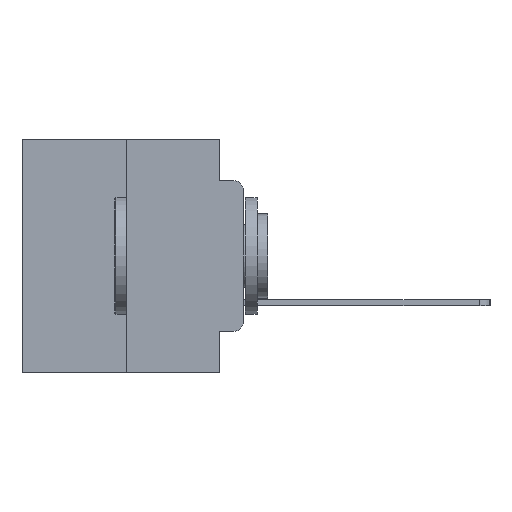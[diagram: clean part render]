
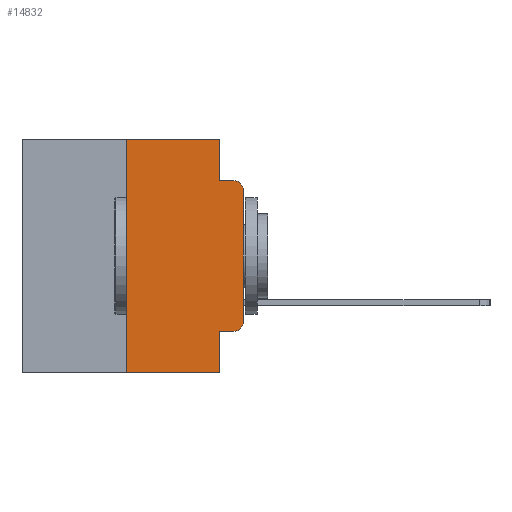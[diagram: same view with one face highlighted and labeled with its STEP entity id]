
A CAD part, left-side view. The second image highlights one B-rep face of the part: STEP entity #14832.
In plain terms, the highlighted planar face has unit normal (-1, 0, 0).
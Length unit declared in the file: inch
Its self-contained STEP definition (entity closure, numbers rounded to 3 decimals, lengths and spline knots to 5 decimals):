
#293 = DIRECTION ( 'NONE',  ( 0., -1., 0. ) ) ;
#563 = DIRECTION ( 'NONE',  ( 0., 0., -1. ) ) ;
#1384 = ORIENTED_EDGE ( 'NONE', *, *, #14961, .F. ) ;
#1643 = LINE ( 'NONE', #5594, #18598 ) ;
#1685 = LINE ( 'NONE', #14650, #23465 ) ;
#1740 = EDGE_CURVE ( 'NONE', #13574, #17665, #1643, .T. ) ;
#1890 = DIRECTION ( 'NONE',  ( 0., -1., 0. ) ) ;
#2057 = VECTOR ( 'NONE', #2701, 39.37008 ) ;
#2079 = CARTESIAN_POINT ( 'NONE',  ( 0., 0.051, -0.4115 ) ) ;
#2270 = CARTESIAN_POINT ( 'NONE',  ( 0., 0., 0. ) ) ;
#2387 = DIRECTION ( 'NONE',  ( 0., -1., 0. ) ) ;
#2701 = DIRECTION ( 'NONE',  ( 0., 0., -1. ) ) ;
#3762 = CARTESIAN_POINT ( 'NONE',  ( 0., 0., -0.1085 ) ) ;
#3891 = DIRECTION ( 'NONE',  ( 0., 0., 1. ) ) ;
#4120 = DIRECTION ( 'NONE',  ( 0., -1., 0. ) ) ;
#4228 = CARTESIAN_POINT ( 'NONE',  ( 0., 0.051, 0. ) ) ;
#4357 = CARTESIAN_POINT ( 'NONE',  ( 0., 0.051, 0. ) ) ;
#5004 = FACE_OUTER_BOUND ( 'NONE', #26360, .T. ) ;
#5014 = ORIENTED_EDGE ( 'NONE', *, *, #18480, .T. ) ;
#5594 = CARTESIAN_POINT ( 'NONE',  ( 0., 0.473, -0.5 ) ) ;
#5695 = ORIENTED_EDGE ( 'NONE', *, *, #17080, .T. ) ;
#5769 = CARTESIAN_POINT ( 'NONE',  ( 0., 0.051, -0.5 ) ) ;
#5929 = VERTEX_POINT ( 'NONE', #19667 ) ;
#6376 = ORIENTED_EDGE ( 'NONE', *, *, #14221, .F. ) ;
#7090 = EDGE_CURVE ( 'NONE', #27107, #26037, #23311, .T. ) ;
#7099 = CARTESIAN_POINT ( 'NONE',  ( 0., 0.02, -0.1085 ) ) ;
#7884 = PLANE ( 'NONE',  #15399 ) ;
#8397 = ORIENTED_EDGE ( 'NONE', *, *, #9958, .F. ) ;
#8549 = EDGE_CURVE ( 'NONE', #12620, #27107, #23541, .T. ) ;
#8835 = AXIS2_PLACEMENT_3D ( 'NONE', #7099, #21842, #9261 ) ;
#9261 = DIRECTION ( 'NONE',  ( 0., 0., -1. ) ) ;
#9958 = EDGE_CURVE ( 'NONE', #12620, #17665, #11955, .T. ) ;
#11428 = VECTOR ( 'NONE', #3891, 39.37008 ) ;
#11955 = LINE ( 'NONE', #4228, #22459 ) ;
#12131 = CARTESIAN_POINT ( 'NONE',  ( 0., 0.473, 0. ) ) ;
#12415 = VECTOR ( 'NONE', #4120, 39.37008 ) ;
#12528 = CARTESIAN_POINT ( 'NONE',  ( 0., 0.25, 0. ) ) ;
#12605 = CARTESIAN_POINT ( 'NONE',  ( 0., 0.02, -0.4115 ) ) ;
#12620 = VERTEX_POINT ( 'NONE', #24255 ) ;
#12792 = EDGE_CURVE ( 'NONE', #13574, #22755, #17098, .T. ) ;
#13329 = DIRECTION ( 'NONE',  ( -1., 0., 0. ) ) ;
#13376 = LINE ( 'NONE', #15489, #2057 ) ;
#13574 = VERTEX_POINT ( 'NONE', #23852 ) ;
#14066 = LINE ( 'NONE', #15180, #19654 ) ;
#14221 = EDGE_CURVE ( 'NONE', #19597, #5929, #13376, .T. ) ;
#14277 = DIRECTION ( 'NONE',  ( 0., 0., -1. ) ) ;
#14650 = CARTESIAN_POINT ( 'NONE',  ( 0., 0.473, 0. ) ) ;
#14832 = ADVANCED_FACE ( 'NONE', ( #5004 ), #7884, .F. ) ;
#14866 = DIRECTION ( 'NONE',  ( 0., 0., -1. ) ) ;
#14961 = EDGE_CURVE ( 'NONE', #22755, #19597, #1685, .T. ) ;
#15180 = CARTESIAN_POINT ( 'NONE',  ( 0., 0.051, -0.0885 ) ) ;
#15399 = AXIS2_PLACEMENT_3D ( 'NONE', #12131, #26707, #14277 ) ;
#15489 = CARTESIAN_POINT ( 'NONE',  ( 0., 0.051, 0. ) ) ;
#15669 = EDGE_CURVE ( 'NONE', #5929, #20698, #14066, .T. ) ;
#17036 = ORIENTED_EDGE ( 'NONE', *, *, #15669, .F. ) ;
#17080 = EDGE_CURVE ( 'NONE', #20389, #20698, #23771, .T. ) ;
#17098 = LINE ( 'NONE', #26942, #11428 ) ;
#17184 = DIRECTION ( 'NONE',  ( 0., 0., 1. ) ) ;
#17665 = VERTEX_POINT ( 'NONE', #5769 ) ;
#18275 = AXIS2_PLACEMENT_3D ( 'NONE', #25791, #13329, #563 ) ;
#18480 = EDGE_CURVE ( 'NONE', #26037, #20389, #19818, .T. ) ;
#18598 = VECTOR ( 'NONE', #293, 39.37008 ) ;
#18994 = ORIENTED_EDGE ( 'NONE', *, *, #1740, .T. ) ;
#19597 = VERTEX_POINT ( 'NONE', #4357 ) ;
#19624 = ORIENTED_EDGE ( 'NONE', *, *, #8549, .T. ) ;
#19654 = VECTOR ( 'NONE', #2387, 39.37008 ) ;
#19667 = CARTESIAN_POINT ( 'NONE',  ( 0., 0.051, -0.0885 ) ) ;
#19818 = LINE ( 'NONE', #2270, #25295 ) ;
#20389 = VERTEX_POINT ( 'NONE', #3762 ) ;
#20698 = VERTEX_POINT ( 'NONE', #21672 ) ;
#21672 = CARTESIAN_POINT ( 'NONE',  ( 0., 0.02, -0.0885 ) ) ;
#21842 = DIRECTION ( 'NONE',  ( -1., 0., 0. ) ) ;
#22459 = VECTOR ( 'NONE', #14866, 39.37008 ) ;
#22755 = VERTEX_POINT ( 'NONE', #12528 ) ;
#23311 = CIRCLE ( 'NONE', #18275, 0.02 ) ;
#23465 = VECTOR ( 'NONE', #1890, 39.37008 ) ;
#23541 = LINE ( 'NONE', #2079, #12415 ) ;
#23771 = CIRCLE ( 'NONE', #8835, 0.02 ) ;
#23804 = CARTESIAN_POINT ( 'NONE',  ( 0., 0., -0.3915 ) ) ;
#23810 = ORIENTED_EDGE ( 'NONE', *, *, #12792, .F. ) ;
#23852 = CARTESIAN_POINT ( 'NONE',  ( 0., 0.25, -0.5 ) ) ;
#24255 = CARTESIAN_POINT ( 'NONE',  ( 0., 0.051, -0.4115 ) ) ;
#25295 = VECTOR ( 'NONE', #17184, 39.37008 ) ;
#25742 = ORIENTED_EDGE ( 'NONE', *, *, #7090, .T. ) ;
#25791 = CARTESIAN_POINT ( 'NONE',  ( 0., 0.02, -0.3915 ) ) ;
#26037 = VERTEX_POINT ( 'NONE', #23804 ) ;
#26360 = EDGE_LOOP ( 'NONE', ( #5014, #5695, #17036, #6376, #1384, #23810, #18994, #8397, #19624, #25742 ) ) ;
#26707 = DIRECTION ( 'NONE',  ( 1., 0., 0. ) ) ;
#26942 = CARTESIAN_POINT ( 'NONE',  ( 0., 0.25, 0. ) ) ;
#27107 = VERTEX_POINT ( 'NONE', #12605 ) ;
